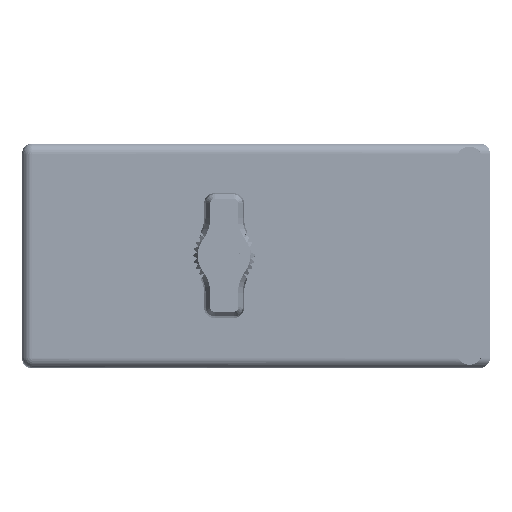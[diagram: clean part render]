
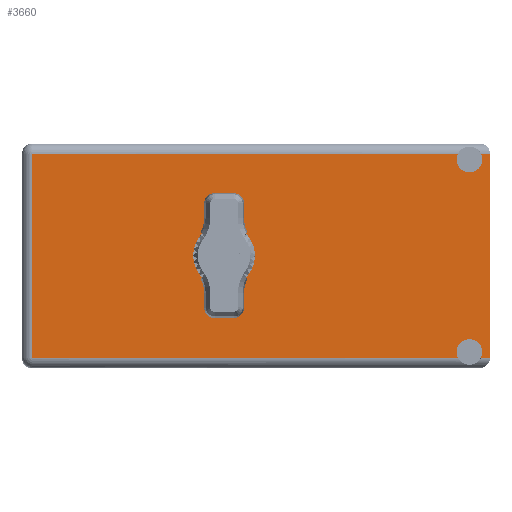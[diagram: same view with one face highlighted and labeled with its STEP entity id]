
A CAD part, top view. The second image highlights one B-rep face of the part: STEP entity #3660.
In plain terms, the highlighted face is planar.
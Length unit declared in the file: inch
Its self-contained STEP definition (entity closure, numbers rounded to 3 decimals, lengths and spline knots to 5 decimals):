
#135 = VERTEX_POINT ( 'NONE', #1800 ) ;
#287 = CIRCLE ( 'NONE', #115076, 0.0875 ) ;
#845 = EDGE_CURVE ( 'NONE', #99327, #63845, #9235, .T. ) ;
#1068 = EDGE_CURVE ( 'NONE', #63845, #99327, #21748, .T. ) ;
#1505 = CARTESIAN_POINT ( 'NONE',  ( -1.3075, 1.93, -0.695 ) ) ;
#1800 = CARTESIAN_POINT ( 'NONE',  ( 1.8125, 1.93, 0.695 ) ) ;
#3603 = CARTESIAN_POINT ( 'NONE',  ( 1.59417, 1.93, 0.695 ) ) ;
#3660 = ADVANCED_FACE ( 'NONE', ( #29688, #46581 ), #58736, .T. ) ;
#3976 = ORIENTED_EDGE ( 'NONE', *, *, #6257, .T. ) ;
#5686 = ORIENTED_EDGE ( 'NONE', *, *, #48419, .F. ) ;
#6257 = EDGE_CURVE ( 'NONE', #26823, #135, #62110, .T. ) ;
#8381 = EDGE_CURVE ( 'NONE', #26823, #92162, #75677, .T. ) ;
#9118 = EDGE_CURVE ( 'NONE', #36612, #135, #107604, .T. ) ;
#9235 = CIRCLE ( 'NONE', #33303, 0.17 ) ;
#10221 = DIRECTION ( 'NONE',  ( 0., 0., 1. ) ) ;
#11210 = DIRECTION ( 'NONE',  ( 0., 1., 0. ) ) ;
#11355 = CARTESIAN_POINT ( 'NONE',  ( 1.75083, 1.93, 0.695 ) ) ;
#12493 = ORIENTED_EDGE ( 'NONE', *, *, #34086, .F. ) ;
#13389 = DIRECTION ( 'NONE',  ( 0., 0., 1. ) ) ;
#13457 = ORIENTED_EDGE ( 'NONE', *, *, #56167, .T. ) ;
#16202 = CIRCLE ( 'NONE', #81702, 0.0875 ) ;
#16372 = CARTESIAN_POINT ( 'NONE',  ( 1.59417, 1.93, -0.695 ) ) ;
#19215 = VECTOR ( 'NONE', #106326, 39.37008 ) ;
#21748 = CIRCLE ( 'NONE', #28154, 0.17 ) ;
#22367 = DIRECTION ( 'NONE',  ( 0., 1., 0. ) ) ;
#25010 = CARTESIAN_POINT ( 'NONE',  ( -1.3775, 1.93, -0.695 ) ) ;
#25386 = CARTESIAN_POINT ( 'NONE',  ( 1.75083, 1.93, -0.695 ) ) ;
#26823 = VERTEX_POINT ( 'NONE', #11355 ) ;
#27977 = DIRECTION ( 'NONE',  ( 0., 0., 1. ) ) ;
#28154 = AXIS2_PLACEMENT_3D ( 'NONE', #44262, #43873, #10221 ) ;
#28241 = AXIS2_PLACEMENT_3D ( 'NONE', #56619, #83210, #31151 ) ;
#29688 = FACE_BOUND ( 'NONE', #102822, .T. ) ;
#31151 = DIRECTION ( 'NONE',  ( 0., 0., 1. ) ) ;
#32142 = CARTESIAN_POINT ( 'NONE',  ( -1.3775, 1.93, -0.765 ) ) ;
#33303 = AXIS2_PLACEMENT_3D ( 'NONE', #67912, #95320, #69097 ) ;
#34086 = EDGE_CURVE ( 'NONE', #53281, #45923, #287, .T. ) ;
#34781 = CARTESIAN_POINT ( 'NONE',  ( 1.8125, 1.93, 0.695 ) ) ;
#36612 = VERTEX_POINT ( 'NONE', #85802 ) ;
#36943 = VECTOR ( 'NONE', #60628, 39.37008 ) ;
#37637 = VECTOR ( 'NONE', #74025, 39.37008 ) ;
#40049 = AXIS2_PLACEMENT_3D ( 'NONE', #32142, #22367, #58335 ) ;
#40261 = CARTESIAN_POINT ( 'NONE',  ( 0., 1.93, 0.17 ) ) ;
#41018 = ORIENTED_EDGE ( 'NONE', *, *, #8381, .F. ) ;
#41908 = VERTEX_POINT ( 'NONE', #1505 ) ;
#43390 = CARTESIAN_POINT ( 'NONE',  ( 1.6725, 1.93, -0.656 ) ) ;
#43873 = DIRECTION ( 'NONE',  ( 0., 1., 0. ) ) ;
#44262 = CARTESIAN_POINT ( 'NONE',  ( 0., 1.93, 0. ) ) ;
#45923 = VERTEX_POINT ( 'NONE', #107536 ) ;
#46581 = FACE_OUTER_BOUND ( 'NONE', #58277, .T. ) ;
#48419 = EDGE_CURVE ( 'NONE', #45923, #79903, #16202, .T. ) ;
#51122 = CIRCLE ( 'NONE', #28241, 0.0875 ) ;
#52891 = VECTOR ( 'NONE', #57100, 39.37008 ) ;
#53281 = VERTEX_POINT ( 'NONE', #16372 ) ;
#55171 = VERTEX_POINT ( 'NONE', #65859 ) ;
#55671 = LINE ( 'NONE', #95492, #52891 ) ;
#56167 = EDGE_CURVE ( 'NONE', #41908, #55171, #71170, .T. ) ;
#56619 = CARTESIAN_POINT ( 'NONE',  ( 1.6725, 1.93, 0.656 ) ) ;
#57100 = DIRECTION ( 'NONE',  ( -1., 0., 0. ) ) ;
#58277 = EDGE_LOOP ( 'NONE', ( #90397, #68406, #41018, #3976, #94507, #60376, #5686, #12493, #83269, #13457 ) ) ;
#58335 = DIRECTION ( 'NONE',  ( -1., 0., 0. ) ) ;
#58736 = PLANE ( 'NONE',  #40049 ) ;
#59680 = CARTESIAN_POINT ( 'NONE',  ( 1.6725, 1.93, -0.656 ) ) ;
#60376 = ORIENTED_EDGE ( 'NONE', *, *, #114887, .T. ) ;
#60628 = DIRECTION ( 'NONE',  ( 1., 0., 0. ) ) ;
#61349 = DIRECTION ( 'NONE',  ( 0., 1., 0. ) ) ;
#62110 = LINE ( 'NONE', #34781, #36943 ) ;
#63845 = VERTEX_POINT ( 'NONE', #40261 ) ;
#64773 = CARTESIAN_POINT ( 'NONE',  ( 1.6725, 1.93, 0.656 ) ) ;
#65859 = CARTESIAN_POINT ( 'NONE',  ( -1.3075, 1.93, 0.695 ) ) ;
#67352 = EDGE_CURVE ( 'NONE', #55171, #91939, #72654, .T. ) ;
#67912 = CARTESIAN_POINT ( 'NONE',  ( 0., 1.93, 0. ) ) ;
#68406 = ORIENTED_EDGE ( 'NONE', *, *, #107122, .F. ) ;
#69097 = DIRECTION ( 'NONE',  ( 0., 0., 1. ) ) ;
#71170 = LINE ( 'NONE', #105002, #106148 ) ;
#72654 = LINE ( 'NONE', #109557, #37637 ) ;
#74025 = DIRECTION ( 'NONE',  ( 1., 0., 0. ) ) ;
#75391 = CARTESIAN_POINT ( 'NONE',  ( 0., 1.93, -0.17 ) ) ;
#75677 = CIRCLE ( 'NONE', #96597, 0.0875 ) ;
#77333 = DIRECTION ( 'NONE',  ( 0., 0., 1. ) ) ;
#78598 = CARTESIAN_POINT ( 'NONE',  ( 1.6725, 1.93, 0.5685 ) ) ;
#78866 = ORIENTED_EDGE ( 'NONE', *, *, #1068, .F. ) ;
#79903 = VERTEX_POINT ( 'NONE', #25386 ) ;
#81702 = AXIS2_PLACEMENT_3D ( 'NONE', #59680, #113612, #77333 ) ;
#83210 = DIRECTION ( 'NONE',  ( 0., 1., 0. ) ) ;
#83269 = ORIENTED_EDGE ( 'NONE', *, *, #115193, .T. ) ;
#85802 = CARTESIAN_POINT ( 'NONE',  ( 1.8125, 1.93, -0.695 ) ) ;
#90397 = ORIENTED_EDGE ( 'NONE', *, *, #67352, .T. ) ;
#90557 = ORIENTED_EDGE ( 'NONE', *, *, #845, .F. ) ;
#91939 = VERTEX_POINT ( 'NONE', #3603 ) ;
#92162 = VERTEX_POINT ( 'NONE', #78598 ) ;
#92780 = CARTESIAN_POINT ( 'NONE',  ( 1.8125, 1.93, 0.765 ) ) ;
#94507 = ORIENTED_EDGE ( 'NONE', *, *, #9118, .F. ) ;
#95320 = DIRECTION ( 'NONE',  ( 0., 1., 0. ) ) ;
#95492 = CARTESIAN_POINT ( 'NONE',  ( -1.3775, 1.93, -0.695 ) ) ;
#96587 = DIRECTION ( 'NONE',  ( 0., 0., 1. ) ) ;
#96597 = AXIS2_PLACEMENT_3D ( 'NONE', #64773, #11210, #27977 ) ;
#96860 = DIRECTION ( 'NONE',  ( 0., 0., 1. ) ) ;
#99327 = VERTEX_POINT ( 'NONE', #75391 ) ;
#102822 = EDGE_LOOP ( 'NONE', ( #78866, #90557 ) ) ;
#103135 = LINE ( 'NONE', #25010, #19215 ) ;
#105002 = CARTESIAN_POINT ( 'NONE',  ( -1.3075, 1.93, -0.765 ) ) ;
#106148 = VECTOR ( 'NONE', #96860, 39.37008 ) ;
#106326 = DIRECTION ( 'NONE',  ( -1., 0., 0. ) ) ;
#107122 = EDGE_CURVE ( 'NONE', #92162, #91939, #51122, .T. ) ;
#107536 = CARTESIAN_POINT ( 'NONE',  ( 1.6725, 1.93, -0.5685 ) ) ;
#107604 = LINE ( 'NONE', #92780, #114728 ) ;
#109557 = CARTESIAN_POINT ( 'NONE',  ( 1.8125, 1.93, 0.695 ) ) ;
#113612 = DIRECTION ( 'NONE',  ( 0., 1., 0. ) ) ;
#114728 = VECTOR ( 'NONE', #13389, 39.37008 ) ;
#114887 = EDGE_CURVE ( 'NONE', #36612, #79903, #55671, .T. ) ;
#115076 = AXIS2_PLACEMENT_3D ( 'NONE', #43390, #61349, #96587 ) ;
#115193 = EDGE_CURVE ( 'NONE', #53281, #41908, #103135, .T. ) ;
